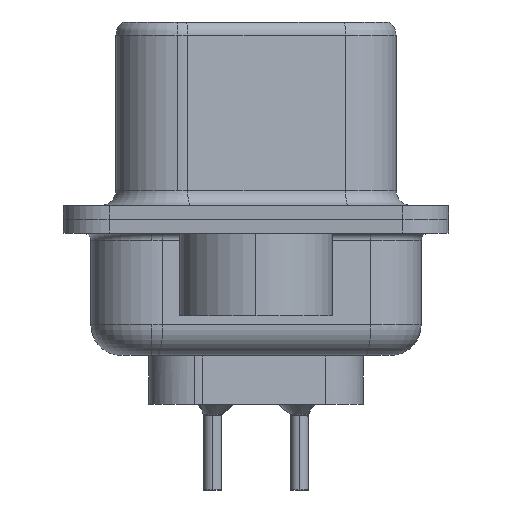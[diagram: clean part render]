
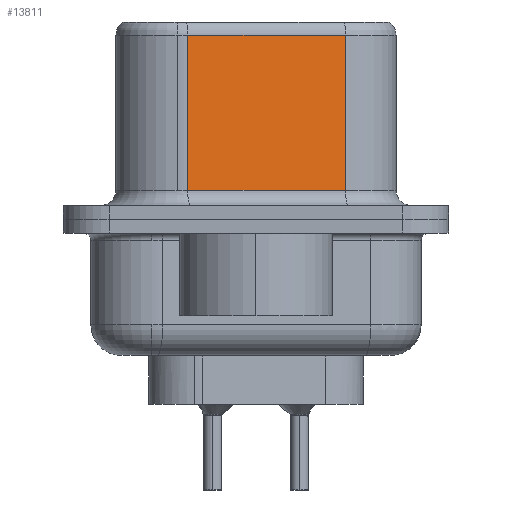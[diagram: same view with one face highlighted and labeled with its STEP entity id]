
A CAD part, left-side view. The second image highlights one B-rep face of the part: STEP entity #13811.
In plain terms, the highlighted planar face has unit normal (-0.985, -0.174, 0).
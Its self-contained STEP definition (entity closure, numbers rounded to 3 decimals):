
#243 = VECTOR ( 'NONE', #15845, 1000. ) ;
#529 = VECTOR ( 'NONE', #7663, 1000. ) ;
#886 = FACE_OUTER_BOUND ( 'NONE', #5081, .T. ) ;
#1024 = PLANE ( 'NONE',  #8425 ) ;
#1746 = EDGE_CURVE ( 'NONE', #14049, #13267, #5092, .T. ) ;
#2079 = EDGE_CURVE ( 'NONE', #6197, #4182, #16885, .T. ) ;
#4182 = VERTEX_POINT ( 'NONE', #14286 ) ;
#4262 = VECTOR ( 'NONE', #15821, 1000. ) ;
#4581 = EDGE_CURVE ( 'NONE', #6197, #14049, #8168, .T. ) ;
#5081 = EDGE_LOOP ( 'NONE', ( #14446, #7262, #5947, #7522 ) ) ;
#5092 = LINE ( 'NONE', #7968, #529 ) ;
#5947 = ORIENTED_EDGE ( 'NONE', *, *, #1746, .T. ) ;
#6197 = VERTEX_POINT ( 'NONE', #7886 ) ;
#7262 = ORIENTED_EDGE ( 'NONE', *, *, #4581, .T. ) ;
#7522 = ORIENTED_EDGE ( 'NONE', *, *, #21423, .T. ) ;
#7663 = DIRECTION ( 'NONE',  ( 0., 0., -1. ) ) ;
#7886 = CARTESIAN_POINT ( 'NONE',  ( 4.575, -2.927, 6.02 ) ) ;
#7968 = CARTESIAN_POINT ( 'NONE',  ( 3.665, 2.233, 6.52 ) ) ;
#8168 = LINE ( 'NONE', #15777, #4262 ) ;
#8425 = AXIS2_PLACEMENT_3D ( 'NONE', #16002, #19200, #9540 ) ;
#9540 = DIRECTION ( 'NONE',  ( -0.174, 0.985, 0. ) ) ;
#12105 = DIRECTION ( 'NONE',  ( 0.174, -0.985, 0. ) ) ;
#13267 = VERTEX_POINT ( 'NONE', #17306 ) ;
#13699 = CARTESIAN_POINT ( 'NONE',  ( 4.575, -2.927, 0.95 ) ) ;
#13811 = ADVANCED_FACE ( 'NONE', ( #886 ), #1024, .F. ) ;
#14049 = VERTEX_POINT ( 'NONE', #16886 ) ;
#14286 = CARTESIAN_POINT ( 'NONE',  ( 4.575, -2.927, 0.95 ) ) ;
#14446 = ORIENTED_EDGE ( 'NONE', *, *, #2079, .F. ) ;
#15455 = VECTOR ( 'NONE', #12105, 1000. ) ;
#15777 = CARTESIAN_POINT ( 'NONE',  ( 4.575, -2.927, 6.02 ) ) ;
#15821 = DIRECTION ( 'NONE',  ( -0.174, 0.985, 0. ) ) ;
#15845 = DIRECTION ( 'NONE',  ( 0., 0., -1. ) ) ;
#16002 = CARTESIAN_POINT ( 'NONE',  ( 4.575, -2.927, 6.52 ) ) ;
#16885 = LINE ( 'NONE', #17606, #243 ) ;
#16886 = CARTESIAN_POINT ( 'NONE',  ( 3.665, 2.233, 6.02 ) ) ;
#17306 = CARTESIAN_POINT ( 'NONE',  ( 3.665, 2.233, 0.95 ) ) ;
#17606 = CARTESIAN_POINT ( 'NONE',  ( 4.575, -2.927, 6.52 ) ) ;
#19200 = DIRECTION ( 'NONE',  ( 0.985, 0.174, 0. ) ) ;
#20198 = LINE ( 'NONE', #13699, #15455 ) ;
#21423 = EDGE_CURVE ( 'NONE', #13267, #4182, #20198, .T. ) ;
